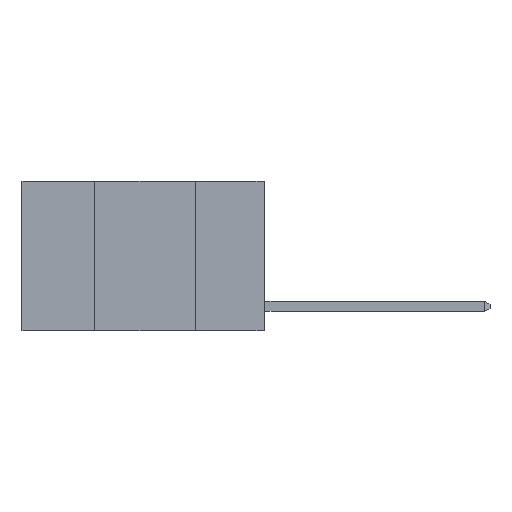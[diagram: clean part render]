
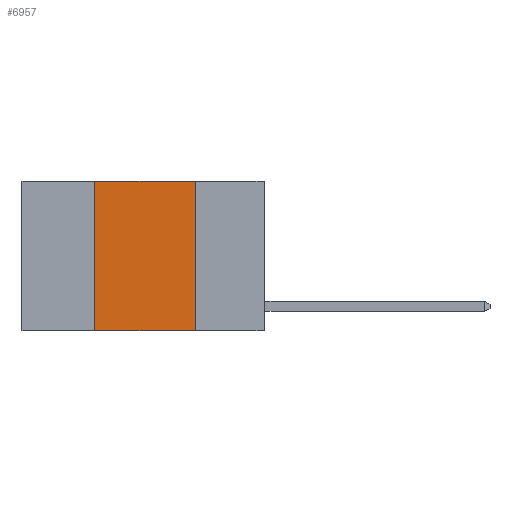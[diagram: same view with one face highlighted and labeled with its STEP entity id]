
A CAD part, left-side view. The second image highlights one B-rep face of the part: STEP entity #6957.
In plain terms, the highlighted planar face has unit normal (-1, 0, 0).
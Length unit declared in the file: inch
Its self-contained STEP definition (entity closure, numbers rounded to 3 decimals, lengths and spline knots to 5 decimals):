
#503 = AXIS2_PLACEMENT_3D ( 'NONE', #8234, #3889, #8947 ) ;
#704 = DIRECTION ( 'NONE',  ( 0., 0., 1. ) ) ;
#719 = CARTESIAN_POINT ( 'NONE',  ( 0., 0.42, 0. ) ) ;
#834 = VERTEX_POINT ( 'NONE', #5869 ) ;
#877 = LINE ( 'NONE', #5235, #6797 ) ;
#1312 = DIRECTION ( 'NONE',  ( 0., -1., 0. ) ) ;
#1460 = PLANE ( 'NONE',  #503 ) ;
#1737 = CARTESIAN_POINT ( 'NONE',  ( 0., 0.17, 0. ) ) ;
#1917 = EDGE_LOOP ( 'NONE', ( #4022, #3971, #3952, #3941 ) ) ;
#2623 = CARTESIAN_POINT ( 'NONE',  ( 0., 0.6, -0.37 ) ) ;
#2952 = DIRECTION ( 'NONE',  ( 0., -1., 0. ) ) ;
#2992 = VERTEX_POINT ( 'NONE', #7980 ) ;
#3071 = VECTOR ( 'NONE', #704, 39.37008 ) ;
#3623 = VECTOR ( 'NONE', #7062, 39.37008 ) ;
#3763 = VERTEX_POINT ( 'NONE', #3870 ) ;
#3870 = CARTESIAN_POINT ( 'NONE',  ( 0., 0.42, -0.37 ) ) ;
#3889 = DIRECTION ( 'NONE',  ( 1., 0., 0. ) ) ;
#3941 = ORIENTED_EDGE ( 'NONE', *, *, #3965, .T. ) ;
#3952 = ORIENTED_EDGE ( 'NONE', *, *, #4292, .F. ) ;
#3965 = EDGE_CURVE ( 'NONE', #3763, #6662, #6162, .T. ) ;
#3971 = ORIENTED_EDGE ( 'NONE', *, *, #9276, .F. ) ;
#4022 = ORIENTED_EDGE ( 'NONE', *, *, #7698, .F. ) ;
#4183 = VECTOR ( 'NONE', #2952, 39.37008 ) ;
#4292 = EDGE_CURVE ( 'NONE', #3763, #834, #7034, .T. ) ;
#4298 = CARTESIAN_POINT ( 'NONE',  ( 0., 0.17, -0.37 ) ) ;
#5235 = CARTESIAN_POINT ( 'NONE',  ( 0., 0.6, 0. ) ) ;
#5869 = CARTESIAN_POINT ( 'NONE',  ( 0., 0.42, 0. ) ) ;
#6162 = LINE ( 'NONE', #2623, #4183 ) ;
#6662 = VERTEX_POINT ( 'NONE', #4298 ) ;
#6797 = VECTOR ( 'NONE', #1312, 39.37008 ) ;
#6890 = FACE_OUTER_BOUND ( 'NONE', #1917, .T. ) ;
#6957 = ADVANCED_FACE ( 'NONE', ( #6890 ), #1460, .F. ) ;
#7034 = LINE ( 'NONE', #719, #3071 ) ;
#7062 = DIRECTION ( 'NONE',  ( 0., 0., -1. ) ) ;
#7698 = EDGE_CURVE ( 'NONE', #2992, #6662, #9182, .T. ) ;
#7980 = CARTESIAN_POINT ( 'NONE',  ( 0., 0.17, 0. ) ) ;
#8234 = CARTESIAN_POINT ( 'NONE',  ( 0., 0.6, 0. ) ) ;
#8947 = DIRECTION ( 'NONE',  ( 0., 0., -1. ) ) ;
#9182 = LINE ( 'NONE', #1737, #3623 ) ;
#9276 = EDGE_CURVE ( 'NONE', #834, #2992, #877, .T. ) ;
